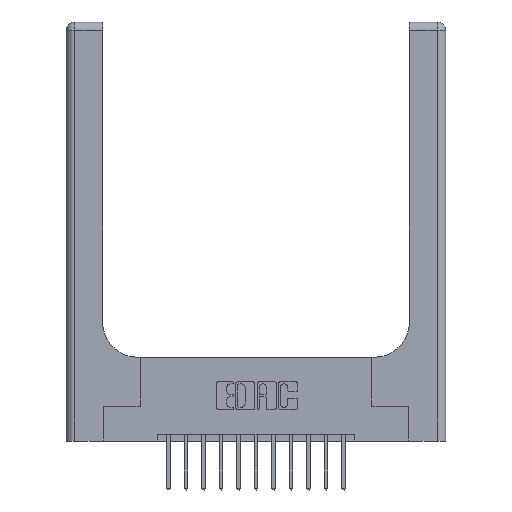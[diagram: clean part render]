
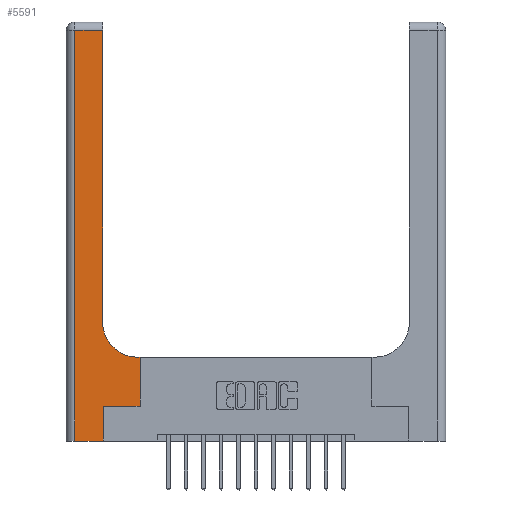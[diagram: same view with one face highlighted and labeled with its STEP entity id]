
A CAD part, top view. The second image highlights one B-rep face of the part: STEP entity #5591.
In plain terms, the highlighted planar face has unit normal (0, 0, 1).
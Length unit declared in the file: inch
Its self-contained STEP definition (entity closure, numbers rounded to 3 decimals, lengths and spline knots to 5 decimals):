
#176 = DIRECTION ( 'NONE',  ( -1., 0., 0. ) ) ;
#403 = CARTESIAN_POINT ( 'NONE',  ( 0.528, 0.25, 0.37 ) ) ;
#417 = VERTEX_POINT ( 'NONE', #15927 ) ;
#825 = VERTEX_POINT ( 'NONE', #8231 ) ;
#888 = VECTOR ( 'NONE', #12595, 39.37008 ) ;
#979 = ORIENTED_EDGE ( 'NONE', *, *, #12615, .T. ) ;
#1566 = CARTESIAN_POINT ( 'NONE',  ( 0., 3., 0.37 ) ) ;
#2013 = EDGE_CURVE ( 'NONE', #825, #7550, #14456, .T. ) ;
#2072 = CARTESIAN_POINT ( 'NONE',  ( 0.51, 0.6, 0.37 ) ) ;
#2631 = CARTESIAN_POINT ( 'NONE',  ( 0.26, 2.94, 0.37 ) ) ;
#2640 = EDGE_CURVE ( 'NONE', #8022, #417, #14825, .T. ) ;
#3526 = CARTESIAN_POINT ( 'NONE',  ( 0., 2.94, 0.37 ) ) ;
#3605 = ORIENTED_EDGE ( 'NONE', *, *, #6524, .T. ) ;
#4118 = DIRECTION ( 'NONE',  ( 0., 0., -1. ) ) ;
#4225 = AXIS2_PLACEMENT_3D ( 'NONE', #1566, #4118, #14374 ) ;
#4360 = ORIENTED_EDGE ( 'NONE', *, *, #5798, .T. ) ;
#4486 = CIRCLE ( 'NONE', #15924, 0.25 ) ;
#4619 = CARTESIAN_POINT ( 'NONE',  ( 0.265, 0., 0.37 ) ) ;
#5096 = ORIENTED_EDGE ( 'NONE', *, *, #11917, .T. ) ;
#5357 = VERTEX_POINT ( 'NONE', #14754 ) ;
#5358 = EDGE_LOOP ( 'NONE', ( #14984, #4360, #3605, #5096, #5879, #979, #12159, #10061, #9087 ) ) ;
#5591 = ADVANCED_FACE ( 'NONE', ( #7949 ), #11684, .F. ) ;
#5634 = DIRECTION ( 'NONE',  ( 0., 0., -1. ) ) ;
#5701 = LINE ( 'NONE', #16425, #888 ) ;
#5798 = EDGE_CURVE ( 'NONE', #12172, #11699, #6720, .T. ) ;
#5813 = DIRECTION ( 'NONE',  ( 0., 1., 0. ) ) ;
#5879 = ORIENTED_EDGE ( 'NONE', *, *, #2640, .T. ) ;
#6092 = VECTOR ( 'NONE', #8625, 39.37008 ) ;
#6208 = CARTESIAN_POINT ( 'NONE',  ( 0.528, 0.25, 0.37 ) ) ;
#6524 = EDGE_CURVE ( 'NONE', #11699, #5357, #5701, .T. ) ;
#6720 = LINE ( 'NONE', #3526, #12718 ) ;
#6757 = VECTOR ( 'NONE', #13569, 39.37008 ) ;
#6772 = EDGE_CURVE ( 'NONE', #7550, #15426, #4486, .T. ) ;
#7328 = VERTEX_POINT ( 'NONE', #403 ) ;
#7385 = CARTESIAN_POINT ( 'NONE',  ( 0.26, 3., 0.37 ) ) ;
#7550 = VERTEX_POINT ( 'NONE', #2072 ) ;
#7696 = EDGE_CURVE ( 'NONE', #7328, #825, #12895, .T. ) ;
#7899 = LINE ( 'NONE', #7385, #11086 ) ;
#7949 = FACE_OUTER_BOUND ( 'NONE', #5358, .T. ) ;
#8013 = CARTESIAN_POINT ( 'NONE',  ( 0.26, 0.6, 0.37 ) ) ;
#8022 = VERTEX_POINT ( 'NONE', #4619 ) ;
#8231 = CARTESIAN_POINT ( 'NONE',  ( 0.528, 0.6, 0.37 ) ) ;
#8305 = CARTESIAN_POINT ( 'NONE',  ( 0.265, 0., 0.37 ) ) ;
#8563 = EDGE_CURVE ( 'NONE', #15426, #12172, #7899, .T. ) ;
#8607 = CARTESIAN_POINT ( 'NONE',  ( 0.06, 2.94, 0.37 ) ) ;
#8625 = DIRECTION ( 'NONE',  ( 0., 1., 0. ) ) ;
#9087 = ORIENTED_EDGE ( 'NONE', *, *, #6772, .T. ) ;
#9292 = CARTESIAN_POINT ( 'NONE',  ( 0.51, 0.85, 0.37 ) ) ;
#9332 = CARTESIAN_POINT ( 'NONE',  ( 0., 0., 0.37 ) ) ;
#10061 = ORIENTED_EDGE ( 'NONE', *, *, #2013, .T. ) ;
#10395 = VECTOR ( 'NONE', #11977, 39.37008 ) ;
#11086 = VECTOR ( 'NONE', #12339, 39.37008 ) ;
#11443 = VECTOR ( 'NONE', #5813, 39.37008 ) ;
#11684 = PLANE ( 'NONE',  #4225 ) ;
#11699 = VERTEX_POINT ( 'NONE', #8607 ) ;
#11917 = EDGE_CURVE ( 'NONE', #5357, #8022, #13780, .T. ) ;
#11945 = DIRECTION ( 'NONE',  ( 1., 0., 0. ) ) ;
#11977 = DIRECTION ( 'NONE',  ( 1., 0., 0. ) ) ;
#12159 = ORIENTED_EDGE ( 'NONE', *, *, #7696, .T. ) ;
#12172 = VERTEX_POINT ( 'NONE', #2631 ) ;
#12339 = DIRECTION ( 'NONE',  ( 0., 1., 0. ) ) ;
#12595 = DIRECTION ( 'NONE',  ( 0., -1., 0. ) ) ;
#12615 = EDGE_CURVE ( 'NONE', #417, #7328, #15356, .T. ) ;
#12718 = VECTOR ( 'NONE', #14938, 39.37008 ) ;
#12895 = LINE ( 'NONE', #6208, #6092 ) ;
#13521 = CARTESIAN_POINT ( 'NONE',  ( 0.265, 0.25, 0.37 ) ) ;
#13569 = DIRECTION ( 'NONE',  ( 1., 0., 0. ) ) ;
#13639 = VECTOR ( 'NONE', #176, 39.37008 ) ;
#13780 = LINE ( 'NONE', #9332, #10395 ) ;
#14374 = DIRECTION ( 'NONE',  ( -1., 0., 0. ) ) ;
#14456 = LINE ( 'NONE', #8013, #13639 ) ;
#14754 = CARTESIAN_POINT ( 'NONE',  ( 0.06, 0., 0.37 ) ) ;
#14825 = LINE ( 'NONE', #8305, #11443 ) ;
#14938 = DIRECTION ( 'NONE',  ( -1., 0., 0. ) ) ;
#14984 = ORIENTED_EDGE ( 'NONE', *, *, #8563, .T. ) ;
#15356 = LINE ( 'NONE', #13521, #6757 ) ;
#15361 = CARTESIAN_POINT ( 'NONE',  ( 0.26, 0.85, 0.37 ) ) ;
#15426 = VERTEX_POINT ( 'NONE', #15361 ) ;
#15924 = AXIS2_PLACEMENT_3D ( 'NONE', #9292, #5634, #11945 ) ;
#15927 = CARTESIAN_POINT ( 'NONE',  ( 0.265, 0.25, 0.37 ) ) ;
#16425 = CARTESIAN_POINT ( 'NONE',  ( 0.06, 3., 0.37 ) ) ;
